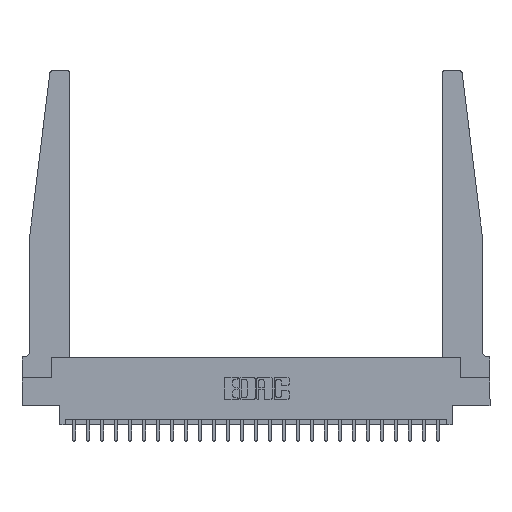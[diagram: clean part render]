
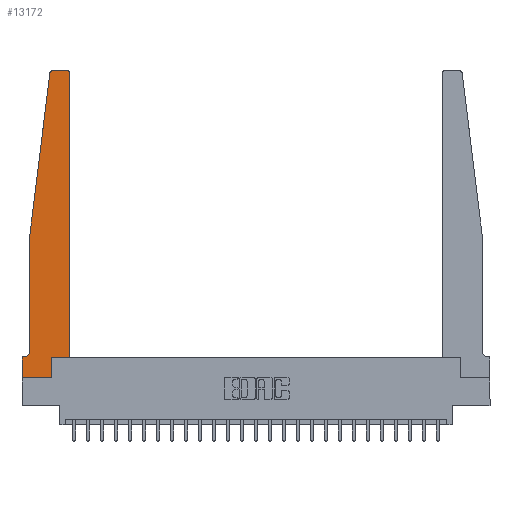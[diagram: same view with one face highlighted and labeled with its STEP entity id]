
A CAD part, top view. The second image highlights one B-rep face of the part: STEP entity #13172.
In plain terms, the highlighted planar face has unit normal (0, 0, 1).
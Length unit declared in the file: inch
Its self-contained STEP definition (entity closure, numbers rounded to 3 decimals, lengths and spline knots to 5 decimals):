
#148 = PLANE ( 'NONE',  #15265 ) ;
#901 = EDGE_CURVE ( 'NONE', #19908, #9550, #19667, .T. ) ;
#1107 = CARTESIAN_POINT ( 'NONE',  ( 0.24675, 2.72367, 0.37 ) ) ;
#1558 = CARTESIAN_POINT ( 'NONE',  ( 0.425, 0.18, 0.37 ) ) ;
#1688 = ORIENTED_EDGE ( 'NONE', *, *, #16389, .T. ) ;
#1707 = DIRECTION ( 'NONE',  ( 1., 0., 0. ) ) ;
#1876 = CARTESIAN_POINT ( 'NONE',  ( 0.065, 1.25, 0.37 ) ) ;
#1903 = DIRECTION ( 'NONE',  ( -1., 0., 0. ) ) ;
#2443 = VERTEX_POINT ( 'NONE', #13906 ) ;
#2473 = VERTEX_POINT ( 'NONE', #7938 ) ;
#2584 = VECTOR ( 'NONE', #9605, 39.37008 ) ;
#3176 = DIRECTION ( 'NONE',  ( 0., 1., 0. ) ) ;
#3345 = CARTESIAN_POINT ( 'NONE',  ( 0.065, 0.1875, 0.37 ) ) ;
#3876 = DIRECTION ( 'NONE',  ( -1., 0., 0. ) ) ;
#3894 = VECTOR ( 'NONE', #16032, 39.37008 ) ;
#4158 = CARTESIAN_POINT ( 'NONE',  ( 0.425, 2.72, 0.37 ) ) ;
#4218 = CARTESIAN_POINT ( 'NONE',  ( 0.27653, 2.75, 0.37 ) ) ;
#5380 = DIRECTION ( 'NONE',  ( 1., 0., 0. ) ) ;
#5414 = EDGE_CURVE ( 'NONE', #8278, #21534, #13796, .T. ) ;
#5459 = CARTESIAN_POINT ( 'NONE',  ( 0.065, 1.25, 0.37 ) ) ;
#5572 = CARTESIAN_POINT ( 'NONE',  ( 0., 0., 0.37 ) ) ;
#6106 = VERTEX_POINT ( 'NONE', #4158 ) ;
#7466 = ORIENTED_EDGE ( 'NONE', *, *, #23236, .T. ) ;
#7513 = CIRCLE ( 'NONE', #24911, 0.05 ) ;
#7636 = CARTESIAN_POINT ( 'NONE',  ( 0.395, 2.72, 0.37 ) ) ;
#7938 = CARTESIAN_POINT ( 'NONE',  ( 0., 0.1875, 0.37 ) ) ;
#7997 = CARTESIAN_POINT ( 'NONE',  ( 0., 0., 0.37 ) ) ;
#8057 = EDGE_CURVE ( 'NONE', #9550, #22293, #7513, .T. ) ;
#8061 = CARTESIAN_POINT ( 'NONE',  ( 0.065, 0.2375, 0.37 ) ) ;
#8278 = VERTEX_POINT ( 'NONE', #19962 ) ;
#8454 = CARTESIAN_POINT ( 'NONE',  ( 0.065, 1.25, 0.37 ) ) ;
#8929 = EDGE_CURVE ( 'NONE', #2473, #15378, #15979, .T. ) ;
#9058 = LINE ( 'NONE', #3345, #15850 ) ;
#9175 = ORIENTED_EDGE ( 'NONE', *, *, #8929, .T. ) ;
#9403 = FACE_OUTER_BOUND ( 'NONE', #11154, .T. ) ;
#9550 = VERTEX_POINT ( 'NONE', #8061 ) ;
#9557 = DIRECTION ( 'NONE',  ( -0.122, -0.992, 0. ) ) ;
#9605 = DIRECTION ( 'NONE',  ( 0., -1., 0. ) ) ;
#9851 = VECTOR ( 'NONE', #21768, 39.37008 ) ;
#10170 = ORIENTED_EDGE ( 'NONE', *, *, #16330, .T. ) ;
#10851 = CARTESIAN_POINT ( 'NONE',  ( 0.425, 0.18, 0.37 ) ) ;
#11154 = EDGE_LOOP ( 'NONE', ( #21419, #7466, #14230, #17237, #19893, #20461, #9175, #23327, #10170, #1688, #11568, #18784 ) ) ;
#11279 = CARTESIAN_POINT ( 'NONE',  ( 0.25, 2.75, 0.37 ) ) ;
#11333 = EDGE_CURVE ( 'NONE', #6106, #8278, #24268, .T. ) ;
#11402 = AXIS2_PLACEMENT_3D ( 'NONE', #15042, #22740, #5380 ) ;
#11568 = ORIENTED_EDGE ( 'NONE', *, *, #16878, .T. ) ;
#11807 = DIRECTION ( 'NONE',  ( 1., 0., 0. ) ) ;
#11823 = DIRECTION ( 'NONE',  ( 1., 0., 0. ) ) ;
#12019 = VECTOR ( 'NONE', #18922, 39.37008 ) ;
#12167 = AXIS2_PLACEMENT_3D ( 'NONE', #7636, #21038, #1707 ) ;
#12875 = VECTOR ( 'NONE', #9557, 39.37008 ) ;
#12883 = CARTESIAN_POINT ( 'NONE',  ( 0.2605, 0.18, 0.37 ) ) ;
#13000 = CIRCLE ( 'NONE', #11402, 0.03 ) ;
#13172 = ADVANCED_FACE ( 'NONE', ( #9403 ), #148, .T. ) ;
#13212 = DIRECTION ( 'NONE',  ( 0., 0., 1. ) ) ;
#13614 = LINE ( 'NONE', #5459, #12875 ) ;
#13796 = LINE ( 'NONE', #11279, #23907 ) ;
#13906 = CARTESIAN_POINT ( 'NONE',  ( 0.425, 0.18, 0.37 ) ) ;
#14230 = ORIENTED_EDGE ( 'NONE', *, *, #15421, .T. ) ;
#14623 = CARTESIAN_POINT ( 'NONE',  ( 0.015, 0.1875, 0.37 ) ) ;
#14633 = LINE ( 'NONE', #10851, #12019 ) ;
#15042 = CARTESIAN_POINT ( 'NONE',  ( 0.27653, 2.72, 0.37 ) ) ;
#15265 = AXIS2_PLACEMENT_3D ( 'NONE', #21389, #13212, #11807 ) ;
#15378 = VERTEX_POINT ( 'NONE', #18657 ) ;
#15421 = EDGE_CURVE ( 'NONE', #23454, #19908, #13614, .T. ) ;
#15615 = LINE ( 'NONE', #5572, #20673 ) ;
#15821 = DIRECTION ( 'NONE',  ( 0., 0., -1. ) ) ;
#15850 = VECTOR ( 'NONE', #22962, 39.37008 ) ;
#15878 = CARTESIAN_POINT ( 'NONE',  ( 0.2605, 0., 0.37 ) ) ;
#15979 = LINE ( 'NONE', #7997, #9851 ) ;
#16032 = DIRECTION ( 'NONE',  ( 0., 1., 0. ) ) ;
#16330 = EDGE_CURVE ( 'NONE', #16646, #23630, #19926, .T. ) ;
#16389 = EDGE_CURVE ( 'NONE', #23630, #2443, #14633, .T. ) ;
#16646 = VERTEX_POINT ( 'NONE', #15878 ) ;
#16878 = EDGE_CURVE ( 'NONE', #2443, #6106, #18886, .T. ) ;
#17237 = ORIENTED_EDGE ( 'NONE', *, *, #901, .T. ) ;
#17281 = VECTOR ( 'NONE', #3176, 39.37008 ) ;
#17346 = CARTESIAN_POINT ( 'NONE',  ( 0.015, 0.2375, 0.37 ) ) ;
#18657 = CARTESIAN_POINT ( 'NONE',  ( 0., 0., 0.37 ) ) ;
#18784 = ORIENTED_EDGE ( 'NONE', *, *, #11333, .T. ) ;
#18886 = LINE ( 'NONE', #1558, #17281 ) ;
#18922 = DIRECTION ( 'NONE',  ( 1., 0., 0. ) ) ;
#19667 = LINE ( 'NONE', #1876, #2584 ) ;
#19893 = ORIENTED_EDGE ( 'NONE', *, *, #8057, .T. ) ;
#19908 = VERTEX_POINT ( 'NONE', #8454 ) ;
#19926 = LINE ( 'NONE', #24115, #3894 ) ;
#19962 = CARTESIAN_POINT ( 'NONE',  ( 0.395, 2.75, 0.37 ) ) ;
#20461 = ORIENTED_EDGE ( 'NONE', *, *, #23736, .T. ) ;
#20673 = VECTOR ( 'NONE', #11823, 39.37008 ) ;
#21038 = DIRECTION ( 'NONE',  ( 0., 0., 1. ) ) ;
#21389 = CARTESIAN_POINT ( 'NONE',  ( 0., 0.1875, 0.37 ) ) ;
#21419 = ORIENTED_EDGE ( 'NONE', *, *, #5414, .T. ) ;
#21534 = VERTEX_POINT ( 'NONE', #4218 ) ;
#21768 = DIRECTION ( 'NONE',  ( 0., -1., 0. ) ) ;
#22293 = VERTEX_POINT ( 'NONE', #14623 ) ;
#22740 = DIRECTION ( 'NONE',  ( 0., 0., 1. ) ) ;
#22962 = DIRECTION ( 'NONE',  ( -1., 0., 0. ) ) ;
#23236 = EDGE_CURVE ( 'NONE', #21534, #23454, #13000, .T. ) ;
#23327 = ORIENTED_EDGE ( 'NONE', *, *, #24187, .T. ) ;
#23454 = VERTEX_POINT ( 'NONE', #1107 ) ;
#23630 = VERTEX_POINT ( 'NONE', #12883 ) ;
#23736 = EDGE_CURVE ( 'NONE', #22293, #2473, #9058, .T. ) ;
#23907 = VECTOR ( 'NONE', #3876, 39.37008 ) ;
#24115 = CARTESIAN_POINT ( 'NONE',  ( 0.2605, 0.18, 0.37 ) ) ;
#24187 = EDGE_CURVE ( 'NONE', #15378, #16646, #15615, .T. ) ;
#24268 = CIRCLE ( 'NONE', #12167, 0.03 ) ;
#24911 = AXIS2_PLACEMENT_3D ( 'NONE', #17346, #15821, #1903 ) ;
